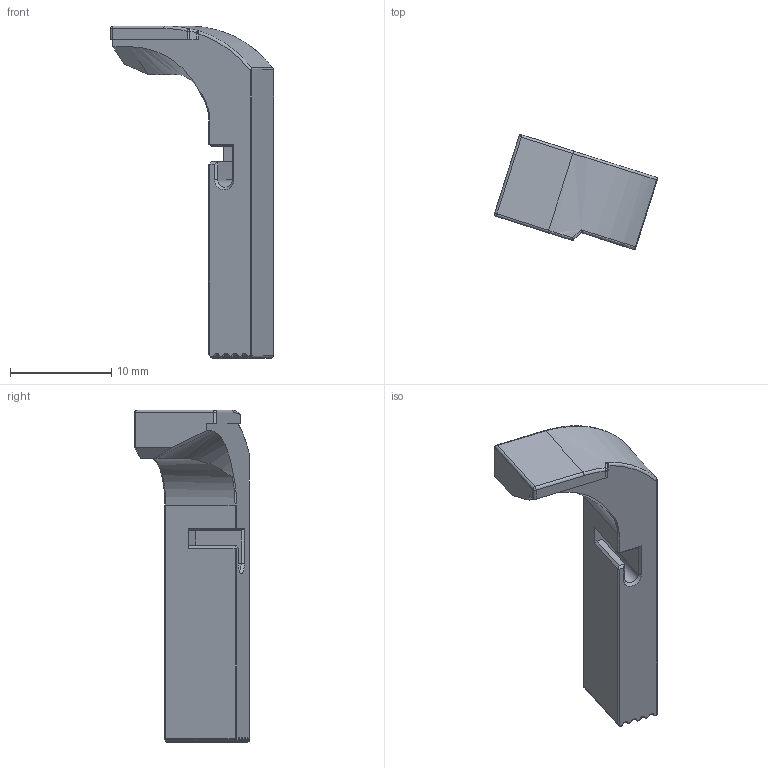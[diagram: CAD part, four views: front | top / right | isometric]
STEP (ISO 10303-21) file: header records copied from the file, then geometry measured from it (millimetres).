
FILE_DESCRIPTION(/* description */ (''),/* implementation_level */ '2;1');
FILE_NAME(/* name */ 'G19 Mag Catch.step',/* time_stamp */ '2019-09-18T22:14:47-04:00',/* author */ (''),/* organization */ (''),/* preprocessor_version */ 'ST-DEVELOPER v18',/* originating_system */ 'Autodesk Translation Framework v8.6.0.1094',/* authorisation */ '');
FILE_SCHEMA (('AUTOMOTIVE_DESIGN { 1 0 10303 214 3 1 1 }'));
Length unit declared in the file: millimetre
Products named in the file (1): Mag Catch
Bounding box: 16.14 x 11.36 x 32.87 mm (x, y, z)
Volume: 1313.4 mm3; surface area: 1071.2 mm2
Topology: 1 solids, 1 shells, 123 faces, 292 edges, 167 vertices
Faces by surface type: cylinder 48, plane 33, bspline 28, torus 10, sphere 3, cone 1
Entity records: 4215 total; most frequent: CARTESIAN_POINT 1441, DIRECTION 578, ORIENTED_EDGE 576, EDGE_CURVE 288, AXIS2_PLACEMENT_3D 222, VERTEX_POINT 167, LINE 134, VECTOR 134
